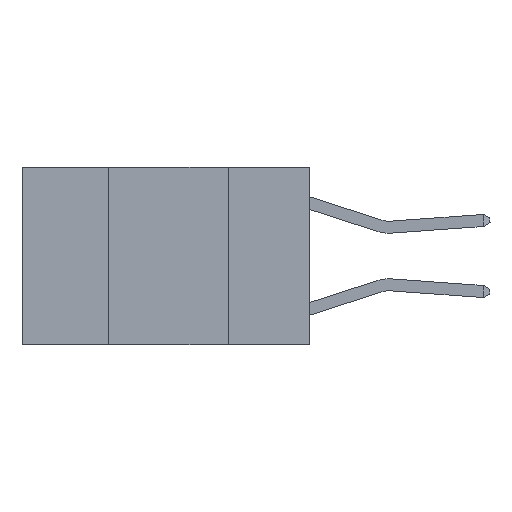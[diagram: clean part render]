
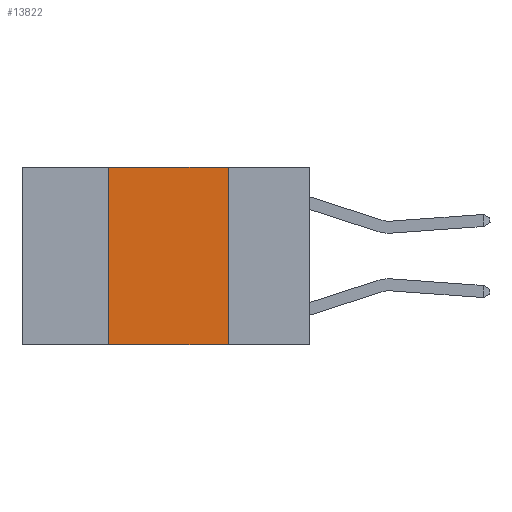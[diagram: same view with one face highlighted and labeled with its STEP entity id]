
A CAD part, left-side view. The second image highlights one B-rep face of the part: STEP entity #13822.
In plain terms, the highlighted planar face has unit normal (-1, 0, 0).
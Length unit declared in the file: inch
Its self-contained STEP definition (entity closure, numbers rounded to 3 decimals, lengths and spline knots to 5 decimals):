
#1258 = CARTESIAN_POINT ( 'NONE',  ( 0., 0.17, 0. ) ) ;
#2105 = VECTOR ( 'NONE', #4422, 39.37008 ) ;
#2979 = VECTOR ( 'NONE', #7889, 39.37008 ) ;
#3411 = CARTESIAN_POINT ( 'NONE',  ( 0., 0.42, 0. ) ) ;
#4422 = DIRECTION ( 'NONE',  ( 0., 0., 1. ) ) ;
#4733 = CARTESIAN_POINT ( 'NONE',  ( 0., 0.17, -0.37 ) ) ;
#4819 = PLANE ( 'NONE',  #15332 ) ;
#5077 = CARTESIAN_POINT ( 'NONE',  ( 0., 0.6, -0.37 ) ) ;
#5137 = VECTOR ( 'NONE', #7264, 39.37008 ) ;
#5286 = FACE_OUTER_BOUND ( 'NONE', #8558, .T. ) ;
#5334 = VERTEX_POINT ( 'NONE', #3411 ) ;
#5543 = LINE ( 'NONE', #8689, #2105 ) ;
#6562 = EDGE_CURVE ( 'NONE', #15047, #11125, #12853, .T. ) ;
#6962 = DIRECTION ( 'NONE',  ( 0., -1., 0. ) ) ;
#7264 = DIRECTION ( 'NONE',  ( 0., 0., -1. ) ) ;
#7336 = ORIENTED_EDGE ( 'NONE', *, *, #11502, .F. ) ;
#7877 = EDGE_CURVE ( 'NONE', #10451, #5334, #5543, .T. ) ;
#7889 = DIRECTION ( 'NONE',  ( 0., -1., 0. ) ) ;
#8558 = EDGE_LOOP ( 'NONE', ( #13481, #7336, #17315, #14594 ) ) ;
#8689 = CARTESIAN_POINT ( 'NONE',  ( 0., 0.42, 0. ) ) ;
#9165 = DIRECTION ( 'NONE',  ( 0., 0., -1. ) ) ;
#9842 = EDGE_CURVE ( 'NONE', #10451, #11125, #11135, .T. ) ;
#10451 = VERTEX_POINT ( 'NONE', #17959 ) ;
#11125 = VERTEX_POINT ( 'NONE', #4733 ) ;
#11135 = LINE ( 'NONE', #5077, #2979 ) ;
#11286 = CARTESIAN_POINT ( 'NONE',  ( 0., 0.6, 0. ) ) ;
#11502 = EDGE_CURVE ( 'NONE', #5334, #15047, #18426, .T. ) ;
#12853 = LINE ( 'NONE', #1258, #5137 ) ;
#13481 = ORIENTED_EDGE ( 'NONE', *, *, #6562, .F. ) ;
#13494 = CARTESIAN_POINT ( 'NONE',  ( 0., 0.6, 0. ) ) ;
#13822 = ADVANCED_FACE ( 'NONE', ( #5286 ), #4819, .F. ) ;
#14594 = ORIENTED_EDGE ( 'NONE', *, *, #9842, .T. ) ;
#14629 = VECTOR ( 'NONE', #6962, 39.37008 ) ;
#15047 = VERTEX_POINT ( 'NONE', #17992 ) ;
#15332 = AXIS2_PLACEMENT_3D ( 'NONE', #13494, #17852, #9165 ) ;
#17315 = ORIENTED_EDGE ( 'NONE', *, *, #7877, .F. ) ;
#17852 = DIRECTION ( 'NONE',  ( 1., 0., 0. ) ) ;
#17959 = CARTESIAN_POINT ( 'NONE',  ( 0., 0.42, -0.37 ) ) ;
#17992 = CARTESIAN_POINT ( 'NONE',  ( 0., 0.17, 0. ) ) ;
#18426 = LINE ( 'NONE', #11286, #14629 ) ;
